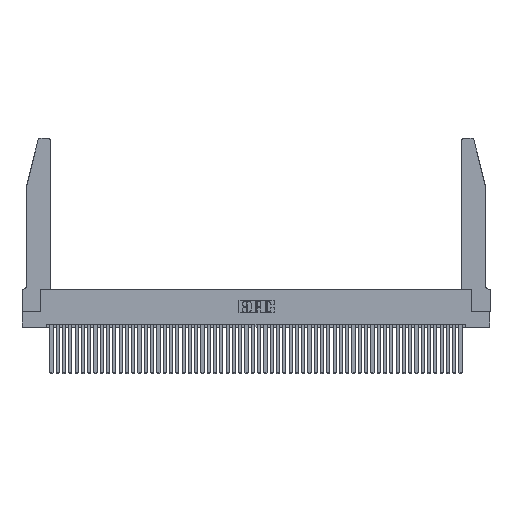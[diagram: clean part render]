
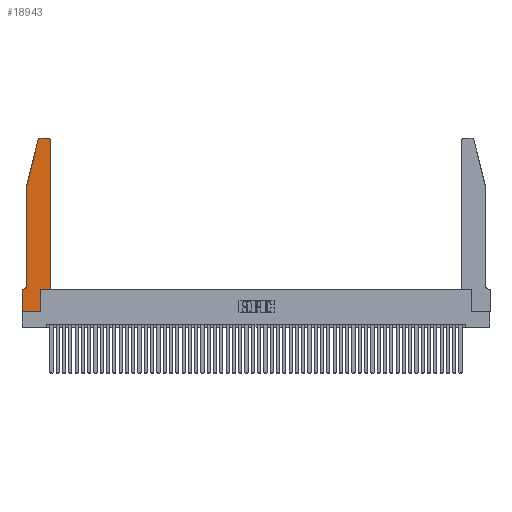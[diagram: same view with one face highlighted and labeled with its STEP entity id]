
A CAD part, top view. The second image highlights one B-rep face of the part: STEP entity #18943.
In plain terms, the highlighted planar face has unit normal (0, 0, 1).
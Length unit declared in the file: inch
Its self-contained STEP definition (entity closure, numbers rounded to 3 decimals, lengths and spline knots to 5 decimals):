
#156 = VECTOR ( 'NONE', #35795, 39.37008 ) ;
#187 = DIRECTION ( 'NONE',  ( 1., 0., 0. ) ) ;
#315 = LINE ( 'NONE', #15631, #1624 ) ;
#1306 = CARTESIAN_POINT ( 'NONE',  ( 0.0755, 2., 0.37 ) ) ;
#1577 = CIRCLE ( 'NONE', #2390, 0.07 ) ;
#1624 = VECTOR ( 'NONE', #19745, 39.37008 ) ;
#2148 = LINE ( 'NONE', #3669, #43274 ) ;
#2390 = AXIS2_PLACEMENT_3D ( 'NONE', #34898, #10269, #39036 ) ;
#2779 = DIRECTION ( 'NONE',  ( -1., 0., 0. ) ) ;
#3448 = VECTOR ( 'NONE', #11630, 39.37008 ) ;
#3495 = DIRECTION ( 'NONE',  ( 1., 0., 0. ) ) ;
#3669 = CARTESIAN_POINT ( 'NONE',  ( 0., 0., 0.37 ) ) ;
#4164 = VERTEX_POINT ( 'NONE', #40319 ) ;
#5477 = DIRECTION ( 'NONE',  ( -0.239, -0.971, 0. ) ) ;
#7735 = EDGE_CURVE ( 'NONE', #27729, #40401, #43554, .T. ) ;
#8218 = DIRECTION ( 'NONE',  ( 0., 0., 1. ) ) ;
#9882 = LINE ( 'NONE', #40427, #18256 ) ;
#9972 = CARTESIAN_POINT ( 'NONE',  ( 0.25487, 2.72718, 0.37 ) ) ;
#10269 = DIRECTION ( 'NONE',  ( 0., 0., -1. ) ) ;
#10600 = EDGE_CURVE ( 'NONE', #50561, #4164, #315, .T. ) ;
#11196 = CARTESIAN_POINT ( 'NONE',  ( 0., 0.35, 0.37 ) ) ;
#11284 = EDGE_CURVE ( 'NONE', #4164, #18502, #14469, .T. ) ;
#11630 = DIRECTION ( 'NONE',  ( 0., -1., 0. ) ) ;
#11718 = EDGE_CURVE ( 'NONE', #31471, #24866, #13120, .T. ) ;
#11769 = EDGE_CURVE ( 'NONE', #24866, #38715, #2148, .T. ) ;
#11777 = AXIS2_PLACEMENT_3D ( 'NONE', #32870, #8218, #36990 ) ;
#12881 = VERTEX_POINT ( 'NONE', #43250 ) ;
#13120 = LINE ( 'NONE', #40371, #3448 ) ;
#13756 = ORIENTED_EDGE ( 'NONE', *, *, #49779, .T. ) ;
#14460 = VECTOR ( 'NONE', #20969, 39.37008 ) ;
#14469 = CIRCLE ( 'NONE', #11777, 0.03 ) ;
#15631 = CARTESIAN_POINT ( 'NONE',  ( 0.2605, 2.75, 0.37 ) ) ;
#15984 = CARTESIAN_POINT ( 'NONE',  ( 0.4205, 2.75, 0.37 ) ) ;
#17948 = VECTOR ( 'NONE', #5477, 39.37008 ) ;
#18256 = VECTOR ( 'NONE', #53028, 39.37008 ) ;
#18502 = VERTEX_POINT ( 'NONE', #9972 ) ;
#18943 = ADVANCED_FACE ( 'NONE', ( #53031 ), #45288, .T. ) ;
#19705 = VERTEX_POINT ( 'NONE', #29304 ) ;
#19745 = DIRECTION ( 'NONE',  ( -1., 0., 0. ) ) ;
#20423 = DIRECTION ( 'NONE',  ( 0., 0., 1. ) ) ;
#20427 = VERTEX_POINT ( 'NONE', #37900 ) ;
#20578 = AXIS2_PLACEMENT_3D ( 'NONE', #20760, #24895, #187 ) ;
#20760 = CARTESIAN_POINT ( 'NONE',  ( 0., 0.35, 0.37 ) ) ;
#20969 = DIRECTION ( 'NONE',  ( 0., 1., 0. ) ) ;
#21502 = ORIENTED_EDGE ( 'NONE', *, *, #11769, .T. ) ;
#21925 = AXIS2_PLACEMENT_3D ( 'NONE', #44967, #20423, #49039 ) ;
#22792 = ORIENTED_EDGE ( 'NONE', *, *, #34736, .T. ) ;
#23318 = CARTESIAN_POINT ( 'NONE',  ( 0.0755, 0.35, 0.37 ) ) ;
#24866 = VERTEX_POINT ( 'NONE', #41556 ) ;
#24895 = DIRECTION ( 'NONE',  ( 0., 0., 1. ) ) ;
#25215 = EDGE_CURVE ( 'NONE', #39149, #20427, #43886, .T. ) ;
#25390 = LINE ( 'NONE', #37315, #14460 ) ;
#27729 = VERTEX_POINT ( 'NONE', #48480 ) ;
#28565 = ORIENTED_EDGE ( 'NONE', *, *, #42478, .T. ) ;
#29075 = EDGE_CURVE ( 'NONE', #12881, #50561, #39134, .T. ) ;
#29304 = CARTESIAN_POINT ( 'NONE',  ( 0.0055, 0.35, 0.37 ) ) ;
#29833 = ORIENTED_EDGE ( 'NONE', *, *, #11718, .T. ) ;
#31370 = LINE ( 'NONE', #23318, #41011 ) ;
#31471 = VERTEX_POINT ( 'NONE', #11196 ) ;
#31658 = CARTESIAN_POINT ( 'NONE',  ( 0.4505, 0.35, 0.37 ) ) ;
#31745 = ORIENTED_EDGE ( 'NONE', *, *, #11284, .T. ) ;
#32870 = CARTESIAN_POINT ( 'NONE',  ( 0.284, 2.72, 0.37 ) ) ;
#33472 = CARTESIAN_POINT ( 'NONE',  ( 0.2865, 0., 0.37 ) ) ;
#34524 = DIRECTION ( 'NONE',  ( 0., -1., 0. ) ) ;
#34736 = EDGE_CURVE ( 'NONE', #38715, #39149, #25390, .T. ) ;
#34898 = CARTESIAN_POINT ( 'NONE',  ( 0.0055, 0.42, 0.37 ) ) ;
#35795 = DIRECTION ( 'NONE',  ( 1., 0., 0. ) ) ;
#36195 = CARTESIAN_POINT ( 'NONE',  ( 0.0755, 0.42, 0.37 ) ) ;
#36990 = DIRECTION ( 'NONE',  ( 1., 0., 0. ) ) ;
#37315 = CARTESIAN_POINT ( 'NONE',  ( 0.2865, 0.35, 0.37 ) ) ;
#37574 = ORIENTED_EDGE ( 'NONE', *, *, #52390, .T. ) ;
#37900 = CARTESIAN_POINT ( 'NONE',  ( 0.4505, 0.35, 0.37 ) ) ;
#38655 = CARTESIAN_POINT ( 'NONE',  ( 0.0755, 2., 0.37 ) ) ;
#38715 = VERTEX_POINT ( 'NONE', #33472 ) ;
#39036 = DIRECTION ( 'NONE',  ( -1., 0., 0. ) ) ;
#39134 = CIRCLE ( 'NONE', #21925, 0.03 ) ;
#39149 = VERTEX_POINT ( 'NONE', #52313 ) ;
#40043 = EDGE_LOOP ( 'NONE', ( #41373, #31745, #13756, #46446, #49001, #28565, #29833, #21502, #22792, #47113, #37574, #41419 ) ) ;
#40319 = CARTESIAN_POINT ( 'NONE',  ( 0.284, 2.75, 0.37 ) ) ;
#40371 = CARTESIAN_POINT ( 'NONE',  ( 0., 0., 0.37 ) ) ;
#40401 = VERTEX_POINT ( 'NONE', #36195 ) ;
#40427 = CARTESIAN_POINT ( 'NONE',  ( 0.4505, 0.35, 0.37 ) ) ;
#41011 = VECTOR ( 'NONE', #2779, 39.37008 ) ;
#41093 = LINE ( 'NONE', #1306, #17948 ) ;
#41373 = ORIENTED_EDGE ( 'NONE', *, *, #10600, .T. ) ;
#41419 = ORIENTED_EDGE ( 'NONE', *, *, #29075, .T. ) ;
#41556 = CARTESIAN_POINT ( 'NONE',  ( 0., 0., 0.37 ) ) ;
#42294 = VECTOR ( 'NONE', #34524, 39.37008 ) ;
#42478 = EDGE_CURVE ( 'NONE', #19705, #31471, #31370, .T. ) ;
#43250 = CARTESIAN_POINT ( 'NONE',  ( 0.4505, 2.72, 0.37 ) ) ;
#43274 = VECTOR ( 'NONE', #3495, 39.37008 ) ;
#43554 = LINE ( 'NONE', #38655, #42294 ) ;
#43886 = LINE ( 'NONE', #31658, #156 ) ;
#44040 = EDGE_CURVE ( 'NONE', #40401, #19705, #1577, .T. ) ;
#44967 = CARTESIAN_POINT ( 'NONE',  ( 0.4205, 2.72, 0.37 ) ) ;
#45288 = PLANE ( 'NONE',  #20578 ) ;
#46446 = ORIENTED_EDGE ( 'NONE', *, *, #7735, .T. ) ;
#47113 = ORIENTED_EDGE ( 'NONE', *, *, #25215, .T. ) ;
#48480 = CARTESIAN_POINT ( 'NONE',  ( 0.0755, 2., 0.37 ) ) ;
#49001 = ORIENTED_EDGE ( 'NONE', *, *, #44040, .T. ) ;
#49039 = DIRECTION ( 'NONE',  ( 1., 0., 0. ) ) ;
#49779 = EDGE_CURVE ( 'NONE', #18502, #27729, #41093, .T. ) ;
#50561 = VERTEX_POINT ( 'NONE', #15984 ) ;
#52313 = CARTESIAN_POINT ( 'NONE',  ( 0.2865, 0.35, 0.37 ) ) ;
#52390 = EDGE_CURVE ( 'NONE', #20427, #12881, #9882, .T. ) ;
#53028 = DIRECTION ( 'NONE',  ( 0., 1., 0. ) ) ;
#53031 = FACE_OUTER_BOUND ( 'NONE', #40043, .T. ) ;
